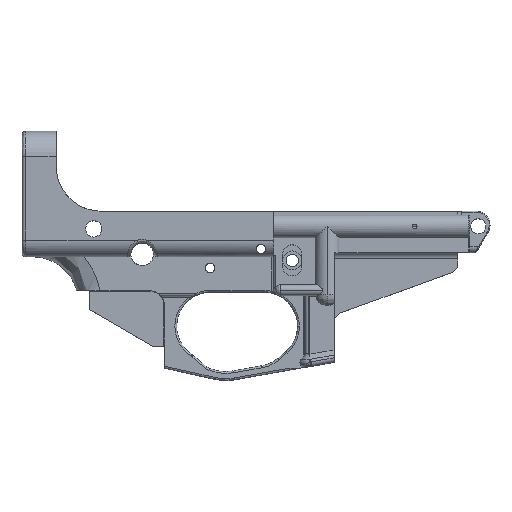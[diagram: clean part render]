
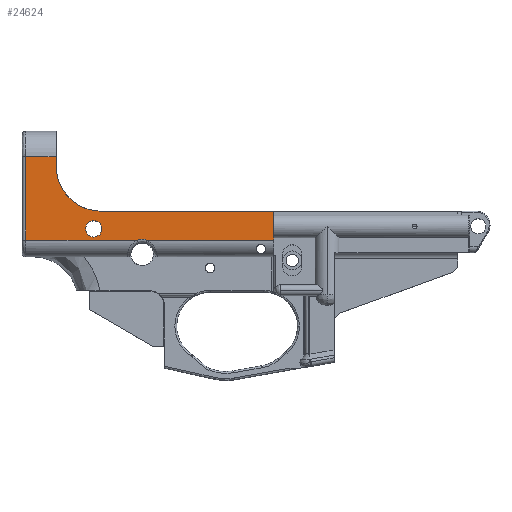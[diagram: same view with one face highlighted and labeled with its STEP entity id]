
A CAD part, top view. The second image highlights one B-rep face of the part: STEP entity #24624.
In plain terms, the highlighted planar face has unit normal (0, 0, 1).
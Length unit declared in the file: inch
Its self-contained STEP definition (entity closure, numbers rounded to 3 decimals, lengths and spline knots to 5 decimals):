
#121 = DIRECTION ( 'NONE',  ( 0., 0., 1. ) ) ;
#198 = CARTESIAN_POINT ( 'NONE',  ( -3.389, -0.22666, 0.73097 ) ) ;
#2272 = EDGE_CURVE ( 'NONE', #10820, #6741, #12302, .T. ) ;
#3408 = DIRECTION ( 'NONE',  ( 1., 0., 0. ) ) ;
#3916 = CARTESIAN_POINT ( 'NONE',  ( -5.49197, -0.22666, 0.73097 ) ) ;
#4330 = AXIS2_PLACEMENT_3D ( 'NONE', #7376, #121, #30809 ) ;
#4343 = DIRECTION ( 'NONE',  ( 1., 0., 0. ) ) ;
#4352 = ORIENTED_EDGE ( 'NONE', *, *, #20315, .F. ) ;
#5153 = LINE ( 'NONE', #8839, #37560 ) ;
#5176 = VECTOR ( 'NONE', #29017, 39.37008 ) ;
#5633 = ORIENTED_EDGE ( 'NONE', *, *, #16011, .F. ) ;
#5652 = AXIS2_PLACEMENT_3D ( 'NONE', #33840, #20090, #30289 ) ;
#6382 = EDGE_CURVE ( 'NONE', #17450, #15523, #16907, .T. ) ;
#6741 = VERTEX_POINT ( 'NONE', #23873 ) ;
#7328 = CARTESIAN_POINT ( 'NONE',  ( -5.51795, -0.21788, 0.73097 ) ) ;
#7376 = CARTESIAN_POINT ( 'NONE',  ( -0.84663, -0.22666, 0.73097 ) ) ;
#7811 = LINE ( 'NONE', #20710, #38076 ) ;
#8307 = CIRCLE ( 'NONE', #22994, 0.135 ) ;
#8839 = CARTESIAN_POINT ( 'NONE',  ( -0.84663, -0.22666, 0.73097 ) ) ;
#8886 = CARTESIAN_POINT ( 'NONE',  ( -7., -0.22666, 0.73097 ) ) ;
#9175 = FACE_OUTER_BOUND ( 'NONE', #12824, .T. ) ;
#9357 = VERTEX_POINT ( 'NONE', #34915 ) ;
#10565 = VERTEX_POINT ( 'NONE', #33581 ) ;
#10616 = CARTESIAN_POINT ( 'NONE',  ( -6.25, 0.2505, 0.73097 ) ) ;
#10795 = DIRECTION ( 'NONE',  ( 0., 1., 0. ) ) ;
#10820 = VERTEX_POINT ( 'NONE', #40266 ) ;
#11091 = CARTESIAN_POINT ( 'NONE',  ( -6.24, -0.0415, 0.73097 ) ) ;
#12015 = ORIENTED_EDGE ( 'NONE', *, *, #2272, .T. ) ;
#12302 = LINE ( 'NONE', #23725, #37218 ) ;
#12652 = CARTESIAN_POINT ( 'NONE',  ( -6.51, -0.0415, 0.73097 ) ) ;
#12824 = EDGE_LOOP ( 'NONE', ( #17832, #15317, #36761, #34104, #12015, #13401, #26422, #17550, #5633 ) ) ;
#13401 = ORIENTED_EDGE ( 'NONE', *, *, #22132, .T. ) ;
#13897 = CARTESIAN_POINT ( 'NONE',  ( -7.5025, -0.22666, 0.73097 ) ) ;
#13907 = CARTESIAN_POINT ( 'NONE',  ( -6.375, -0.0415, 0.73097 ) ) ;
#14305 = CARTESIAN_POINT ( 'NONE',  ( -5.59938, -0.2135, 0.73097 ) ) ;
#15138 = VERTEX_POINT ( 'NONE', #11091 ) ;
#15290 = EDGE_CURVE ( 'NONE', #9357, #29647, #5153, .T. ) ;
#15317 = ORIENTED_EDGE ( 'NONE', *, *, #6382, .T. ) ;
#15380 = VECTOR ( 'NONE', #10795, 39.37008 ) ;
#15523 = VERTEX_POINT ( 'NONE', #36435 ) ;
#16011 = EDGE_CURVE ( 'NONE', #22101, #18216, #7811, .T. ) ;
#16907 = LINE ( 'NONE', #8886, #5176 ) ;
#17450 = VERTEX_POINT ( 'NONE', #32245 ) ;
#17550 = ORIENTED_EDGE ( 'NONE', *, *, #33548, .T. ) ;
#17717 = CARTESIAN_POINT ( 'NONE',  ( -5.62607, -0.21789, 0.73097 ) ) ;
#17787 = EDGE_CURVE ( 'NONE', #22101, #17450, #22080, .T. ) ;
#17832 = ORIENTED_EDGE ( 'NONE', *, *, #17787, .T. ) ;
#18216 = VERTEX_POINT ( 'NONE', #18364 ) ;
#18364 = CARTESIAN_POINT ( 'NONE',  ( -3.389, 0.2505, 0.73097 ) ) ;
#20090 = DIRECTION ( 'NONE',  ( 0., 0., -1. ) ) ;
#20315 = EDGE_CURVE ( 'NONE', #31559, #15138, #39038, .T. ) ;
#20682 = VECTOR ( 'NONE', #32046, 39.37008 ) ;
#20710 = CARTESIAN_POINT ( 'NONE',  ( 0., 0.2505, 0.73097 ) ) ;
#20809 = LINE ( 'NONE', #13897, #26113 ) ;
#20925 = DIRECTION ( 'NONE',  ( 1., 0., 0. ) ) ;
#21144 = CARTESIAN_POINT ( 'NONE',  ( -5.65203, -0.22666, 0.73097 ) ) ;
#21323 = CARTESIAN_POINT ( 'NONE',  ( -3.389, 0., 0.73097 ) ) ;
#22080 = CIRCLE ( 'NONE', #5652, 0.75 ) ;
#22101 = VERTEX_POINT ( 'NONE', #10616 ) ;
#22132 = EDGE_CURVE ( 'NONE', #6741, #9357, #34998, .T. ) ;
#22994 = AXIS2_PLACEMENT_3D ( 'NONE', #34552, #24884, #20925 ) ;
#23725 = CARTESIAN_POINT ( 'NONE',  ( -0.84663, -0.22666, 0.73097 ) ) ;
#23873 = CARTESIAN_POINT ( 'NONE',  ( -5.65203, -0.22666, 0.73097 ) ) ;
#24240 = CARTESIAN_POINT ( 'NONE',  ( -5.54462, -0.2135, 0.73097 ) ) ;
#24624 = ADVANCED_FACE ( 'NONE', ( #30910, #9175 ), #41019, .T. ) ;
#24884 = DIRECTION ( 'NONE',  ( 0., 0., 1. ) ) ;
#25094 = EDGE_CURVE ( 'NONE', #10565, #10820, #20809, .T. ) ;
#26113 = VECTOR ( 'NONE', #41151, 39.37008 ) ;
#26422 = ORIENTED_EDGE ( 'NONE', *, *, #15290, .T. ) ;
#29017 = DIRECTION ( 'NONE',  ( 0., 1., 0. ) ) ;
#29647 = VERTEX_POINT ( 'NONE', #198 ) ;
#30289 = DIRECTION ( 'NONE',  ( 1., 0., 0. ) ) ;
#30809 = DIRECTION ( 'NONE',  ( 1., 0., 0. ) ) ;
#30910 = FACE_BOUND ( 'NONE', #33692, .T. ) ;
#31559 = VERTEX_POINT ( 'NONE', #12652 ) ;
#32046 = DIRECTION ( 'NONE',  ( -1., 0., 0. ) ) ;
#32245 = CARTESIAN_POINT ( 'NONE',  ( -7., 1.0005, 0.73097 ) ) ;
#33326 = ORIENTED_EDGE ( 'NONE', *, *, #37716, .F. ) ;
#33548 = EDGE_CURVE ( 'NONE', #29647, #18216, #43498, .T. ) ;
#33581 = CARTESIAN_POINT ( 'NONE',  ( -7.5025, 1.15661, 0.73097 ) ) ;
#33692 = EDGE_LOOP ( 'NONE', ( #4352, #33326 ) ) ;
#33840 = CARTESIAN_POINT ( 'NONE',  ( -6.25, 1.0005, 0.73097 ) ) ;
#34104 = ORIENTED_EDGE ( 'NONE', *, *, #25094, .T. ) ;
#34187 = EDGE_CURVE ( 'NONE', #15523, #10565, #42939, .T. ) ;
#34552 = CARTESIAN_POINT ( 'NONE',  ( -6.375, -0.0415, 0.73097 ) ) ;
#34915 = CARTESIAN_POINT ( 'NONE',  ( -5.49197, -0.22666, 0.73097 ) ) ;
#34998 = B_SPLINE_CURVE_WITH_KNOTS ( 'NONE', 3,
 ( #21144, #17717, #14305, #24240, #7328, #3916 ),
 .UNSPECIFIED., .F., .F.,
 ( 4, 2, 4 ),
 ( 0., 0.5, 1. ),
 .UNSPECIFIED. ) ;
#36435 = CARTESIAN_POINT ( 'NONE',  ( -7., 1.15661, 0.73097 ) ) ;
#36761 = ORIENTED_EDGE ( 'NONE', *, *, #34187, .T. ) ;
#37218 = VECTOR ( 'NONE', #3408, 39.37008 ) ;
#37560 = VECTOR ( 'NONE', #41594, 39.37008 ) ;
#37630 = DIRECTION ( 'NONE',  ( 1., 0., 0. ) ) ;
#37716 = EDGE_CURVE ( 'NONE', #15138, #31559, #8307, .T. ) ;
#37774 = DIRECTION ( 'NONE',  ( 0., 0., 1. ) ) ;
#38076 = VECTOR ( 'NONE', #4343, 39.37008 ) ;
#39038 = CIRCLE ( 'NONE', #39847, 0.135 ) ;
#39847 = AXIS2_PLACEMENT_3D ( 'NONE', #13907, #37774, #37630 ) ;
#40266 = CARTESIAN_POINT ( 'NONE',  ( -7.5025, -0.22666, 0.73097 ) ) ;
#41019 = PLANE ( 'NONE',  #4330 ) ;
#41151 = DIRECTION ( 'NONE',  ( 0., -1., 0. ) ) ;
#41594 = DIRECTION ( 'NONE',  ( 1., 0., 0. ) ) ;
#42252 = CARTESIAN_POINT ( 'NONE',  ( -0.84663, 1.15661, 0.73097 ) ) ;
#42939 = LINE ( 'NONE', #42252, #20682 ) ;
#43498 = LINE ( 'NONE', #21323, #15380 ) ;
